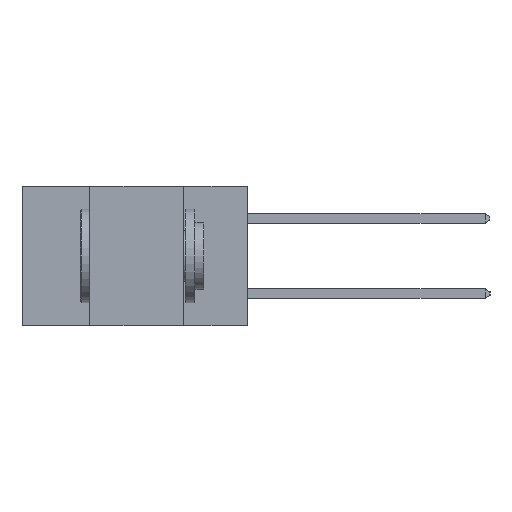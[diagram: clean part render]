
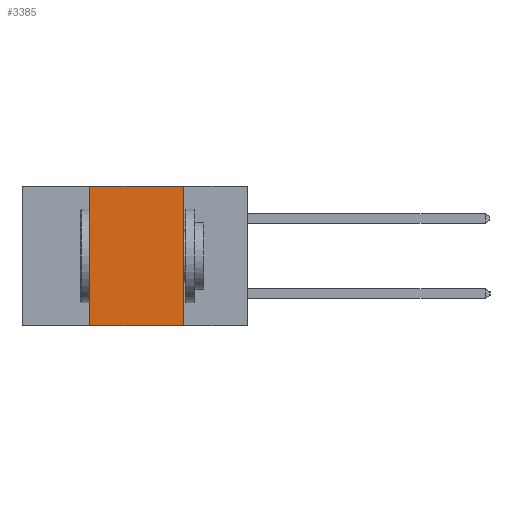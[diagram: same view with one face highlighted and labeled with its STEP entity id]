
A CAD part, left-side view. The second image highlights one B-rep face of the part: STEP entity #3385.
In plain terms, the highlighted planar face has unit normal (-1, 0, 0).
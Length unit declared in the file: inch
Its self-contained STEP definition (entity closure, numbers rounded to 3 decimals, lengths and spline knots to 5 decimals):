
#599 = CARTESIAN_POINT ( 'NONE',  ( 0., 0.42, -0.37 ) ) ;
#790 = VECTOR ( 'NONE', #11384, 39.37008 ) ;
#854 = LINE ( 'NONE', #11416, #5718 ) ;
#1846 = PLANE ( 'NONE',  #11014 ) ;
#2551 = LINE ( 'NONE', #6782, #9653 ) ;
#2586 = ORIENTED_EDGE ( 'NONE', *, *, #11125, .F. ) ;
#2772 = ORIENTED_EDGE ( 'NONE', *, *, #11693, .F. ) ;
#2812 = CARTESIAN_POINT ( 'NONE',  ( 0., 0.6, 0. ) ) ;
#3385 = ADVANCED_FACE ( 'NONE', ( #11055 ), #1846, .F. ) ;
#4087 = CARTESIAN_POINT ( 'NONE',  ( 0., 0.17, -0.37 ) ) ;
#5033 = LINE ( 'NONE', #5184, #790 ) ;
#5184 = CARTESIAN_POINT ( 'NONE',  ( 0., 0.42, -0.37 ) ) ;
#5718 = VECTOR ( 'NONE', #6178, 39.37008 ) ;
#5775 = DIRECTION ( 'NONE',  ( 0., 0., -1. ) ) ;
#5967 = VERTEX_POINT ( 'NONE', #4087 ) ;
#6178 = DIRECTION ( 'NONE',  ( 0., -1., 0. ) ) ;
#6733 = VECTOR ( 'NONE', #11794, 39.37008 ) ;
#6782 = CARTESIAN_POINT ( 'NONE',  ( 0., 0.6, 0. ) ) ;
#7581 = CARTESIAN_POINT ( 'NONE',  ( 0., 0.42, 0. ) ) ;
#7670 = VERTEX_POINT ( 'NONE', #599 ) ;
#8155 = EDGE_CURVE ( 'NONE', #7670, #5967, #854, .T. ) ;
#9063 = LINE ( 'NONE', #10954, #6733 ) ;
#9653 = VECTOR ( 'NONE', #11153, 39.37008 ) ;
#10217 = ORIENTED_EDGE ( 'NONE', *, *, #8155, .T. ) ;
#10327 = VERTEX_POINT ( 'NONE', #7581 ) ;
#10368 = ORIENTED_EDGE ( 'NONE', *, *, #10556, .F. ) ;
#10525 = EDGE_LOOP ( 'NONE', ( #2772, #2586, #10368, #10217 ) ) ;
#10556 = EDGE_CURVE ( 'NONE', #7670, #10327, #5033, .T. ) ;
#10954 = CARTESIAN_POINT ( 'NONE',  ( 0., 0.17, -0.37 ) ) ;
#11014 = AXIS2_PLACEMENT_3D ( 'NONE', #2812, #11039, #5775 ) ;
#11039 = DIRECTION ( 'NONE',  ( 1., 0., 0. ) ) ;
#11055 = FACE_OUTER_BOUND ( 'NONE', #10525, .T. ) ;
#11060 = VERTEX_POINT ( 'NONE', #11078 ) ;
#11078 = CARTESIAN_POINT ( 'NONE',  ( 0., 0.17, 0. ) ) ;
#11125 = EDGE_CURVE ( 'NONE', #10327, #11060, #2551, .T. ) ;
#11153 = DIRECTION ( 'NONE',  ( 0., -1., 0. ) ) ;
#11384 = DIRECTION ( 'NONE',  ( 0., 0., 1. ) ) ;
#11416 = CARTESIAN_POINT ( 'NONE',  ( 0., 0.6, -0.37 ) ) ;
#11693 = EDGE_CURVE ( 'NONE', #11060, #5967, #9063, .T. ) ;
#11794 = DIRECTION ( 'NONE',  ( 0., 0., -1. ) ) ;
